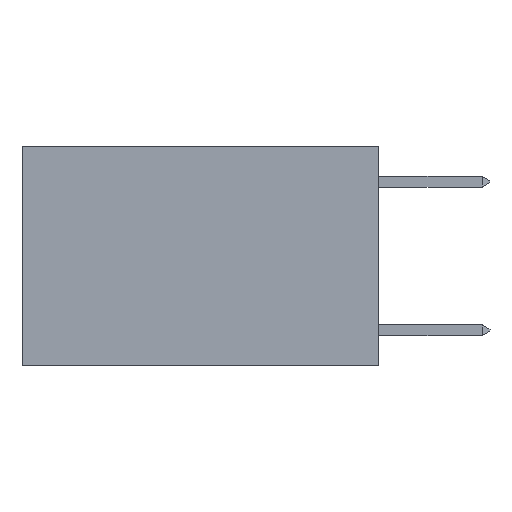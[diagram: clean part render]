
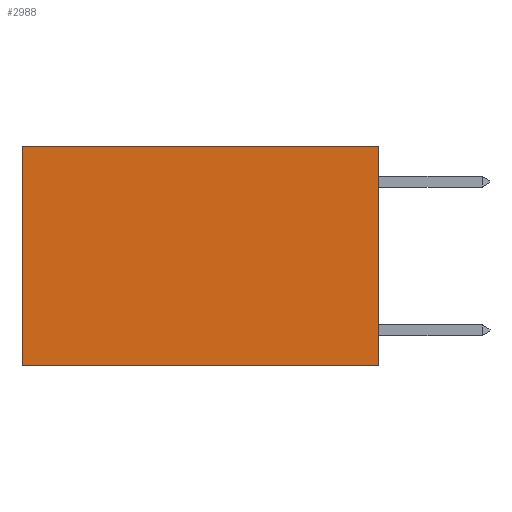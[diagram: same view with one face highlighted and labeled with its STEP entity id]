
A CAD part, left-side view. The second image highlights one B-rep face of the part: STEP entity #2988.
In plain terms, the highlighted planar face has unit normal (-1, 0, 0).
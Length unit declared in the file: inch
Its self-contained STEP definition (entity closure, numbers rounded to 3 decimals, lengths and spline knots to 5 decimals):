
#561 = EDGE_CURVE ( 'NONE', #4399, #8288, #7899, .T. ) ;
#1018 = EDGE_CURVE ( 'NONE', #8288, #7546, #8263, .T. ) ;
#1191 = AXIS2_PLACEMENT_3D ( 'NONE', #2246, #7003, #8205 ) ;
#1361 = CARTESIAN_POINT ( 'NONE',  ( 0.2625, 0.6, -0.37 ) ) ;
#1381 = CARTESIAN_POINT ( 'NONE',  ( 0.2625, 0., -0.37 ) ) ;
#1712 = VECTOR ( 'NONE', #9525, 39.37008 ) ;
#2246 = CARTESIAN_POINT ( 'NONE',  ( 0.2625, 0., 0. ) ) ;
#2328 = CARTESIAN_POINT ( 'NONE',  ( 0.2625, 0., 0. ) ) ;
#2988 = ADVANCED_FACE ( 'NONE', ( #7107 ), #4437, .F. ) ;
#3099 = DIRECTION ( 'NONE',  ( 0., 0., -1. ) ) ;
#3304 = VECTOR ( 'NONE', #8310, 39.37008 ) ;
#3682 = DIRECTION ( 'NONE',  ( 0., 1., 0. ) ) ;
#4399 = VERTEX_POINT ( 'NONE', #4729 ) ;
#4437 = PLANE ( 'NONE',  #1191 ) ;
#4491 = CARTESIAN_POINT ( 'NONE',  ( 0.2625, 0., 0. ) ) ;
#4729 = CARTESIAN_POINT ( 'NONE',  ( 0.2625, 0., 0. ) ) ;
#4857 = EDGE_CURVE ( 'NONE', #4399, #9043, #6236, .T. ) ;
#5463 = ORIENTED_EDGE ( 'NONE', *, *, #4857, .T. ) ;
#5790 = CARTESIAN_POINT ( 'NONE',  ( 0.2625, 0.6, 0. ) ) ;
#5821 = ORIENTED_EDGE ( 'NONE', *, *, #1018, .F. ) ;
#6236 = LINE ( 'NONE', #4491, #10077 ) ;
#6450 = ORIENTED_EDGE ( 'NONE', *, *, #561, .F. ) ;
#7003 = DIRECTION ( 'NONE',  ( 1., 0., 0. ) ) ;
#7107 = FACE_OUTER_BOUND ( 'NONE', #8800, .T. ) ;
#7513 = CARTESIAN_POINT ( 'NONE',  ( 0.2625, 0.6, 0. ) ) ;
#7546 = VERTEX_POINT ( 'NONE', #1361 ) ;
#7899 = LINE ( 'NONE', #2328, #9691 ) ;
#7983 = ORIENTED_EDGE ( 'NONE', *, *, #8509, .T. ) ;
#8205 = DIRECTION ( 'NONE',  ( 0., 0., -1. ) ) ;
#8263 = LINE ( 'NONE', #9551, #1712 ) ;
#8288 = VERTEX_POINT ( 'NONE', #1381 ) ;
#8310 = DIRECTION ( 'NONE',  ( 0., 0., -1. ) ) ;
#8509 = EDGE_CURVE ( 'NONE', #9043, #7546, #9677, .T. ) ;
#8800 = EDGE_LOOP ( 'NONE', ( #7983, #5821, #6450, #5463 ) ) ;
#9043 = VERTEX_POINT ( 'NONE', #5790 ) ;
#9525 = DIRECTION ( 'NONE',  ( 0., 1., 0. ) ) ;
#9551 = CARTESIAN_POINT ( 'NONE',  ( 0.2625, 0., -0.37 ) ) ;
#9677 = LINE ( 'NONE', #7513, #3304 ) ;
#9691 = VECTOR ( 'NONE', #3099, 39.37008 ) ;
#10077 = VECTOR ( 'NONE', #3682, 39.37008 ) ;
